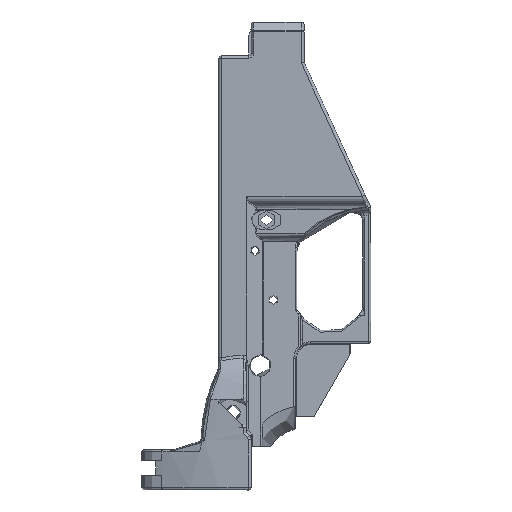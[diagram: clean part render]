
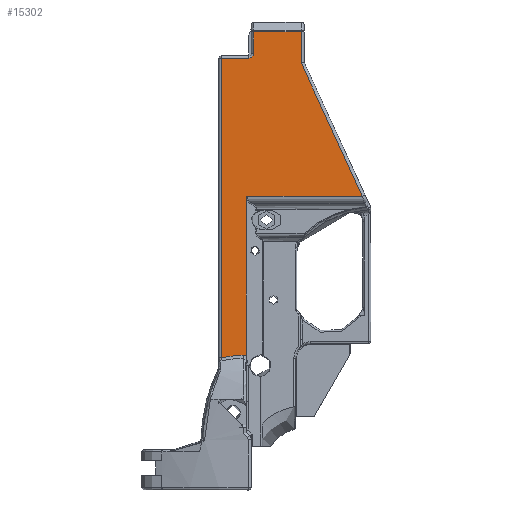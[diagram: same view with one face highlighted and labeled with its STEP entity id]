
A CAD part, left-side view. The second image highlights one B-rep face of the part: STEP entity #15302.
In plain terms, the highlighted planar face has unit normal (-1, 0, 0).
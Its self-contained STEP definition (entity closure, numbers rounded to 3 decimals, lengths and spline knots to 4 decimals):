
#221=ELLIPSE('',#16680,1.9201,1.636);
#399=PLANE('',#16678);
#1321=FACE_OUTER_BOUND('',#2277,.T.);
#2277=EDGE_LOOP('',(#12157,#12158,#12159,#12160,#12161,#12162,#12163,#12164,
#12165,#12166,#12167,#12168));
#3185=B_SPLINE_CURVE_WITH_KNOTS('',3,(#42403,#42404,#42405,#42406),
 .UNSPECIFIED.,.F.,.F.,(4,4),(-0.1434,0.),
 .UNSPECIFIED.);
#3186=B_SPLINE_CURVE_WITH_KNOTS('',3,(#42410,#42411,#42412,#42413,#42414,
#42415,#42416,#42417,#42418,#42419,#42420,#42421),.UNSPECIFIED.,.F.,.F.,
(4,2,2,2,2,4),(-0.117,-0.1147,-0.0798,
-0.057,-0.0072,0.),.UNSPECIFIED.);
#3819=CIRCLE('',#16679,0.08);
#4477=LINE('',#25062,#5245);
#4479=LINE('',#25093,#5247);
#4660=LINE('',#42355,#5428);
#4664=LINE('',#42393,#5432);
#4665=LINE('',#42397,#5433);
#4666=LINE('',#42399,#5434);
#4667=LINE('',#42408,#5435);
#4668=LINE('',#42422,#5436);
#5245=VECTOR('',#18820,0.3937);
#5247=VECTOR('',#18832,0.3937);
#5428=VECTOR('',#19681,0.3937);
#5432=VECTOR('',#19703,0.3937);
#5433=VECTOR('',#19706,0.3937);
#5434=VECTOR('',#19707,0.3937);
#5435=VECTOR('',#19710,1.6985);
#5436=VECTOR('',#19711,0.1181);
#6211=VERTEX_POINT('',#25059);
#6212=VERTEX_POINT('',#25061);
#6216=VERTEX_POINT('',#25091);
#6686=VERTEX_POINT('',#42353);
#6691=VERTEX_POINT('',#42392);
#6692=VERTEX_POINT('',#42394);
#6693=VERTEX_POINT('',#42396);
#6694=VERTEX_POINT('',#42398);
#6695=VERTEX_POINT('',#42400);
#6696=VERTEX_POINT('',#42402);
#6697=VERTEX_POINT('',#42407);
#6698=VERTEX_POINT('',#42409);
#7928=EDGE_CURVE('',#6211,#6212,#4477,.T.);
#7935=EDGE_CURVE('',#6216,#6211,#4479,.T.);
#8638=EDGE_CURVE('',#6686,#6216,#4660,.T.);
#8647=EDGE_CURVE('',#6691,#6686,#4664,.T.);
#8648=EDGE_CURVE('',#6692,#6691,#3819,.T.);
#8649=EDGE_CURVE('',#6693,#6692,#4665,.T.);
#8650=EDGE_CURVE('',#6694,#6693,#4666,.T.);
#8651=EDGE_CURVE('',#6695,#6694,#221,.T.);
#8652=EDGE_CURVE('',#6696,#6695,#3185,.T.);
#8653=EDGE_CURVE('',#6697,#6696,#4667,.T.);
#8654=EDGE_CURVE('',#6698,#6697,#3186,.T.);
#8655=EDGE_CURVE('',#6212,#6698,#4668,.T.);
#12157=ORIENTED_EDGE('',*,*,#7928,.F.);
#12158=ORIENTED_EDGE('',*,*,#7935,.F.);
#12159=ORIENTED_EDGE('',*,*,#8638,.F.);
#12160=ORIENTED_EDGE('',*,*,#8647,.F.);
#12161=ORIENTED_EDGE('',*,*,#8648,.F.);
#12162=ORIENTED_EDGE('',*,*,#8649,.F.);
#12163=ORIENTED_EDGE('',*,*,#8650,.F.);
#12164=ORIENTED_EDGE('',*,*,#8651,.F.);
#12165=ORIENTED_EDGE('',*,*,#8652,.F.);
#12166=ORIENTED_EDGE('',*,*,#8653,.F.);
#12167=ORIENTED_EDGE('',*,*,#8654,.F.);
#12168=ORIENTED_EDGE('',*,*,#8655,.F.);
#15302=ADVANCED_FACE('',(#1321),#399,.F.);
#16678=AXIS2_PLACEMENT_3D('',#42391,#19701,#19702);
#16679=AXIS2_PLACEMENT_3D('',#42395,#19704,#19705);
#16680=AXIS2_PLACEMENT_3D('',#42401,#19708,#19709);
#18820=DIRECTION('',(0.,-0.417,-0.909));
#18832=DIRECTION('',(0.,0.,-1.));
#19681=DIRECTION('',(0.,-1.,0.));
#19701=DIRECTION('center_axis',(1.,0.,0.));
#19702=DIRECTION('ref_axis',(0.,0.,
-1.));
#19703=DIRECTION('',(0.,0.,1.));
#19704=DIRECTION('center_axis',(-1.,0.,0.));
#19705=DIRECTION('ref_axis',(0.,-0.707,-0.707));
#19706=DIRECTION('',(0.,-1.,0.));
#19707=DIRECTION('',(0.,0.,1.));
#19708=DIRECTION('center_axis',(-1.,0.,0.));
#19709=DIRECTION('ref_axis',(0.,-0.984,-0.179));
#19710=DIRECTION('',(0.,0.,-1.));
#19711=DIRECTION('',(0.,1.,0.));
#25059=CARTESIAN_POINT('',(-0.731,-0.0727,2.8507));
#25061=CARTESIAN_POINT('',(-0.731,-1.118,0.5717));
#25062=CARTESIAN_POINT('',(-0.731,-1.4648,-0.1846));
#25091=CARTESIAN_POINT('',(-0.731,-0.0728,3.3816));
#25093=CARTESIAN_POINT('',(-0.731,-0.0727,-0.2092));
#42353=CARTESIAN_POINT('',(-0.731,0.7372,3.3816));
#42355=CARTESIAN_POINT('',(-0.731,0.7121,3.3816));
#42391=CARTESIAN_POINT('Origin',(-0.731,0.68,-3.6849));
#42392=CARTESIAN_POINT('',(-0.731,0.7373,3.0095));
#42393=CARTESIAN_POINT('',(-0.731,0.7373,-0.0118));
#42394=CARTESIAN_POINT('',(-0.731,0.8173,2.9295));
#42395=CARTESIAN_POINT('Origin',(-0.731,0.8173,3.0095));
#42396=CARTESIAN_POINT('',(-0.731,1.2902,2.9295));
#42397=CARTESIAN_POINT('',(-0.731,0.7441,2.9295));
#42398=CARTESIAN_POINT('',(-0.731,1.2902,-2.1813));
#42399=CARTESIAN_POINT('',(-0.731,1.2902,-3.1756));
#42400=CARTESIAN_POINT('',(-0.731,0.9158,-2.1342));
#42401=CARTESIAN_POINT('Origin',(-0.731,0.7244,-3.7785));
#42402=CARTESIAN_POINT('',(-0.731,0.8628,-2.151));
#42403=CARTESIAN_POINT('Ctrl Pts',(-0.731,0.8629,
-2.151));
#42404=CARTESIAN_POINT('Ctrl Pts',(-0.731,0.8784,
-2.1404));
#42405=CARTESIAN_POINT('Ctrl Pts',(-0.731,0.8969,
-2.1335));
#42406=CARTESIAN_POINT('Ctrl Pts',(-0.731,0.9158,
-2.1342));
#42407=CARTESIAN_POINT('',(-0.731,0.8628,0.5319));
#42408=CARTESIAN_POINT('',(-0.731,0.8628,-2.5001));
#42409=CARTESIAN_POINT('',(-0.731,0.8546,0.5717));
#42410=CARTESIAN_POINT('Ctrl Pts',(-0.731,0.8546,
0.5717));
#42411=CARTESIAN_POINT('Ctrl Pts',(-0.731,0.8546,
0.5716));
#42412=CARTESIAN_POINT('Ctrl Pts',(-0.731,0.8546,
0.5716));
#42413=CARTESIAN_POINT('Ctrl Pts',(-0.731,0.855,
0.5706));
#42414=CARTESIAN_POINT('Ctrl Pts',(-0.731,0.8564,
0.5674));
#42415=CARTESIAN_POINT('Ctrl Pts',(-0.731,0.8587,
0.5601));
#42416=CARTESIAN_POINT('Ctrl Pts',(-0.731,0.8595,
0.5572));
#42417=CARTESIAN_POINT('Ctrl Pts',(-0.731,0.8617,
0.5478));
#42418=CARTESIAN_POINT('Ctrl Pts',(-0.731,0.8626,
0.5413));
#42419=CARTESIAN_POINT('Ctrl Pts',(-0.731,0.8628,
0.5338));
#42420=CARTESIAN_POINT('Ctrl Pts',(-0.731,0.8628,
0.5329));
#42421=CARTESIAN_POINT('Ctrl Pts',(-0.731,0.8628,
0.5319));
#42422=CARTESIAN_POINT('',(-0.731,1.0895,0.5717));
